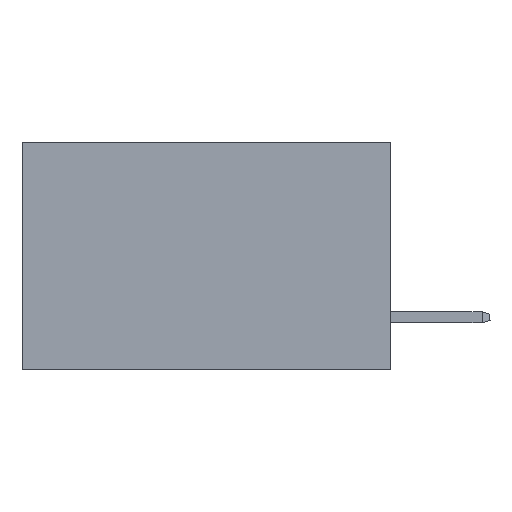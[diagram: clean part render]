
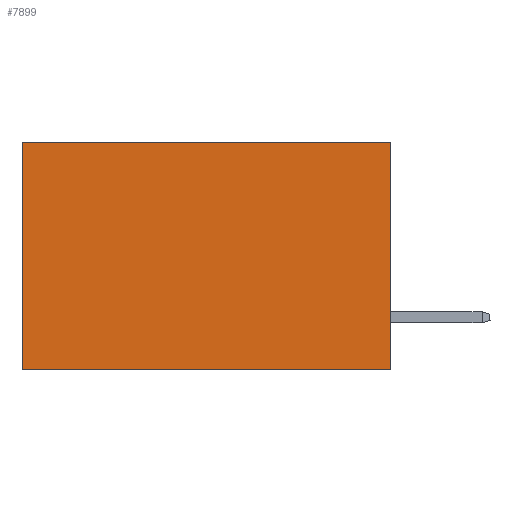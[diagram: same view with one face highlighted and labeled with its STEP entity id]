
A CAD part, left-side view. The second image highlights one B-rep face of the part: STEP entity #7899.
In plain terms, the highlighted planar face has unit normal (-1, 0, 0).
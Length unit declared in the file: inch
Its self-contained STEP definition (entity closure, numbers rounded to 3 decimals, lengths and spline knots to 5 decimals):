
#281 = DIRECTION ( 'NONE',  ( 0., 1., 0. ) ) ;
#627 = DIRECTION ( 'NONE',  ( 0., 0., -1. ) ) ;
#1496 = VECTOR ( 'NONE', #7887, 39.37008 ) ;
#2144 = CARTESIAN_POINT ( 'NONE',  ( 0.2875, 0., 0. ) ) ;
#2542 = AXIS2_PLACEMENT_3D ( 'NONE', #6526, #12526, #627 ) ;
#2733 = VECTOR ( 'NONE', #6255, 39.37008 ) ;
#3820 = VERTEX_POINT ( 'NONE', #8279 ) ;
#4045 = ORIENTED_EDGE ( 'NONE', *, *, #6739, .F. ) ;
#4077 = LINE ( 'NONE', #2144, #4248 ) ;
#4248 = VECTOR ( 'NONE', #7193, 39.37008 ) ;
#4570 = VECTOR ( 'NONE', #281, 39.37008 ) ;
#4681 = FACE_OUTER_BOUND ( 'NONE', #7738, .T. ) ;
#5233 = VERTEX_POINT ( 'NONE', #10079 ) ;
#5252 = EDGE_CURVE ( 'NONE', #3820, #5233, #8988, .T. ) ;
#6255 = DIRECTION ( 'NONE',  ( 0., 0., -1. ) ) ;
#6279 = CARTESIAN_POINT ( 'NONE',  ( 0.2875, 0., -0.37 ) ) ;
#6385 = EDGE_CURVE ( 'NONE', #7246, #3820, #6768, .T. ) ;
#6526 = CARTESIAN_POINT ( 'NONE',  ( 0.2875, 0., 0. ) ) ;
#6739 = EDGE_CURVE ( 'NONE', #7574, #5233, #9120, .T. ) ;
#6768 = LINE ( 'NONE', #8604, #1496 ) ;
#7045 = CARTESIAN_POINT ( 'NONE',  ( 0.2875, 0., 0. ) ) ;
#7052 = ORIENTED_EDGE ( 'NONE', *, *, #6385, .T. ) ;
#7193 = DIRECTION ( 'NONE',  ( 0., 0., -1. ) ) ;
#7213 = CARTESIAN_POINT ( 'NONE',  ( 0.2875, 0.6, 0. ) ) ;
#7246 = VERTEX_POINT ( 'NONE', #7045 ) ;
#7574 = VERTEX_POINT ( 'NONE', #6279 ) ;
#7738 = EDGE_LOOP ( 'NONE', ( #12266, #4045, #8733, #7052 ) ) ;
#7887 = DIRECTION ( 'NONE',  ( 0., 1., 0. ) ) ;
#7899 = ADVANCED_FACE ( 'NONE', ( #4681 ), #10617, .F. ) ;
#7939 = EDGE_CURVE ( 'NONE', #7246, #7574, #4077, .T. ) ;
#8279 = CARTESIAN_POINT ( 'NONE',  ( 0.2875, 0.6, 0. ) ) ;
#8604 = CARTESIAN_POINT ( 'NONE',  ( 0.2875, 0., 0. ) ) ;
#8733 = ORIENTED_EDGE ( 'NONE', *, *, #7939, .F. ) ;
#8988 = LINE ( 'NONE', #7213, #2733 ) ;
#9120 = LINE ( 'NONE', #10095, #4570 ) ;
#10079 = CARTESIAN_POINT ( 'NONE',  ( 0.2875, 0.6, -0.37 ) ) ;
#10095 = CARTESIAN_POINT ( 'NONE',  ( 0.2875, 0., -0.37 ) ) ;
#10617 = PLANE ( 'NONE',  #2542 ) ;
#12266 = ORIENTED_EDGE ( 'NONE', *, *, #5252, .T. ) ;
#12526 = DIRECTION ( 'NONE',  ( 1., 0., 0. ) ) ;
